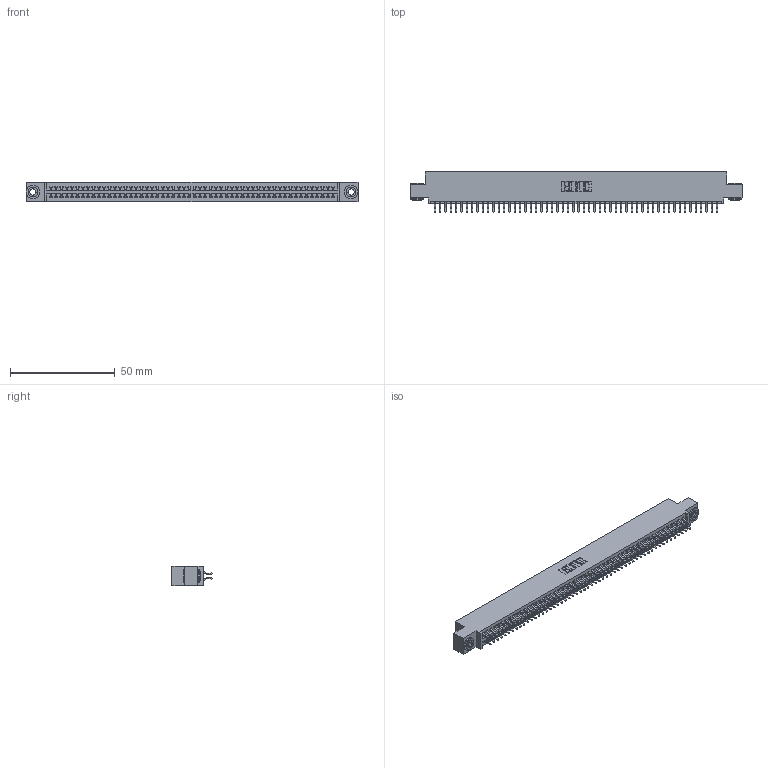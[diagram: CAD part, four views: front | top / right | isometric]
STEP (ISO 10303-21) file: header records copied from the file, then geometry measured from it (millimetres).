
FILE_DESCRIPTION (( 'STEP AP203' ), '1' );
FILE_NAME ('395-108-556-503.STEP', '2018-11-30T23:35:01', ( '' ), ( '' ), 'SwSTEP 2.0', 'SolidWorks 2016', '' );
FILE_SCHEMA (( 'CONFIG_CONTROL_DESIGN' ));
Length unit declared in the file: inch
Products named in the file (4): 345 Part_0.110 Offset - 0.156 Dia-TH; 345-250-002_345-250-002-102; 345-292-001_556 Tail; 395-108-556-503
Assembly tree (111 placements, depth 2):
  395-108-556-503
    345 Part_0.110 Offset - 0.156 Dia-TH
    345-292-001_556 Tail  x108
    345-250-002_345-250-002-102  x2
Bounding box: 158.37 x 19.24 x 9.4 mm (x, y, z)
Volume: 15437.3 mm3; surface area: 23254.5 mm2
Topology: 111 solids, 111 shells, 6216 faces, 18465 edges, 12162 vertices
Faces by surface type: plane 4090, cylinder 2118, cone 8
Entity records: 41756 total; most frequent: CARTESIAN_POINT 6979, ORIENTED_EDGE 6894, DIRECTION 6157, EDGE_CURVE 3447, LINE 3067, VECTOR 3067, VERTEX_POINT 2294, AXIS2_PLACEMENT_3D 1545
